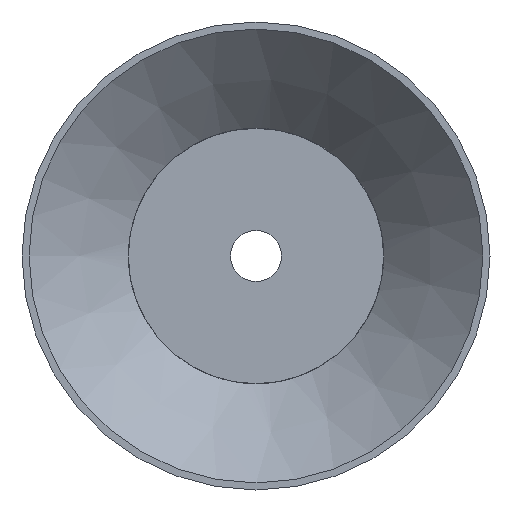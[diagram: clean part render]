
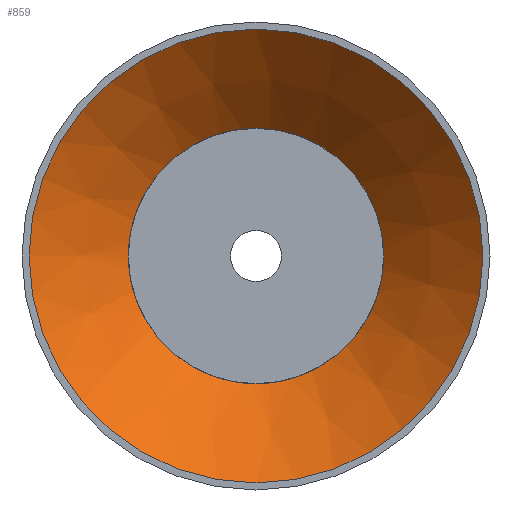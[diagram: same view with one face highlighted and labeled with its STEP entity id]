
A CAD part, front view. The second image highlights one B-rep face of the part: STEP entity #859.
In plain terms, the highlighted conical face has half-angle 45.227 degrees and reference radius 31.679 mm.
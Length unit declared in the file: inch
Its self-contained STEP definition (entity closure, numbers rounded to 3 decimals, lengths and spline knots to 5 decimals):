
#100=(
BOUNDED_CURVE()
B_SPLINE_CURVE(2,(#1197,#1198,#1199),.UNSPECIFIED.,.F.,.F.)
B_SPLINE_CURVE_WITH_KNOTS((3,3),(0.,0.0225),.UNSPECIFIED.)
CURVE()
GEOMETRIC_REPRESENTATION_ITEM()
RATIONAL_B_SPLINE_CURVE((1.,1.,1.))
REPRESENTATION_ITEM('')
);
#101=(
BOUNDED_CURVE()
B_SPLINE_CURVE(2,(#1201,#1202,#1203),.UNSPECIFIED.,.F.,.F.)
B_SPLINE_CURVE_WITH_KNOTS((3,3),(0.84945,0.87196),
 .UNSPECIFIED.)
CURVE()
GEOMETRIC_REPRESENTATION_ITEM()
RATIONAL_B_SPLINE_CURVE((1.,1.,1.))
REPRESENTATION_ITEM('')
);
#102=(
BOUNDED_CURVE()
B_SPLINE_CURVE(2,(#1206,#1207,#1208),.UNSPECIFIED.,.F.,.F.)
B_SPLINE_CURVE_WITH_KNOTS((3,3),(0.,0.0225),.UNSPECIFIED.)
CURVE()
GEOMETRIC_REPRESENTATION_ITEM()
RATIONAL_B_SPLINE_CURVE((1.,1.,1.))
REPRESENTATION_ITEM('')
);
#103=(
BOUNDED_CURVE()
B_SPLINE_CURVE(2,(#1210,#1211,#1212),.UNSPECIFIED.,.F.,.F.)
B_SPLINE_CURVE_WITH_KNOTS((3,3),(0.84929,0.87179),
 .UNSPECIFIED.)
CURVE()
GEOMETRIC_REPRESENTATION_ITEM()
RATIONAL_B_SPLINE_CURVE((1.,1.,1.))
REPRESENTATION_ITEM('')
);
#104=(
BOUNDED_CURVE()
B_SPLINE_CURVE(2,(#1215,#1216,#1217),.UNSPECIFIED.,.F.,.F.)
B_SPLINE_CURVE_WITH_KNOTS((3,3),(0.,0.0225),.UNSPECIFIED.)
CURVE()
GEOMETRIC_REPRESENTATION_ITEM()
RATIONAL_B_SPLINE_CURVE((1.,1.,1.))
REPRESENTATION_ITEM('')
);
#105=(
BOUNDED_CURVE()
B_SPLINE_CURVE(2,(#1219,#1220,#1221),.UNSPECIFIED.,.F.,.F.)
B_SPLINE_CURVE_WITH_KNOTS((3,3),(0.84951,0.87201),
 .UNSPECIFIED.)
CURVE()
GEOMETRIC_REPRESENTATION_ITEM()
RATIONAL_B_SPLINE_CURVE((1.,1.,1.))
REPRESENTATION_ITEM('')
);
#106=(
BOUNDED_CURVE()
B_SPLINE_CURVE(2,(#1224,#1225,#1226),.UNSPECIFIED.,.F.,.F.)
B_SPLINE_CURVE_WITH_KNOTS((3,3),(0.,0.0225),.UNSPECIFIED.)
CURVE()
GEOMETRIC_REPRESENTATION_ITEM()
RATIONAL_B_SPLINE_CURVE((1.,1.,1.))
REPRESENTATION_ITEM('')
);
#107=(
BOUNDED_CURVE()
B_SPLINE_CURVE(2,(#1228,#1229,#1230),.UNSPECIFIED.,.F.,.F.)
B_SPLINE_CURVE_WITH_KNOTS((3,3),(0.8493,0.8718),
 .UNSPECIFIED.)
CURVE()
GEOMETRIC_REPRESENTATION_ITEM()
RATIONAL_B_SPLINE_CURVE((1.,1.,1.))
REPRESENTATION_ITEM('')
);
#128=CONICAL_SURFACE('',#932,1.24721,0.789);
#137=FACE_OUTER_BOUND('',#178,.T.);
#178=EDGE_LOOP('',(#588,#589,#590,#591,#592,#593,#594,#595,#596,#597,#598,
#599,#600,#601,#602,#603,#604,#605,#606,#607,#608));
#223=LINE('',#1194,#253);
#253=VECTOR('',#1037,1.24721);
#279=CIRCLE('',#915,0.89443);
#280=CIRCLE('',#917,0.89443);
#282=CIRCLE('',#920,0.89443);
#285=CIRCLE('',#924,0.89443);
#289=CIRCLE('',#930,1.6);
#290=CIRCLE('',#931,1.6);
#291=CIRCLE('',#933,0.9);
#292=CIRCLE('',#934,0.9);
#293=CIRCLE('',#935,0.9);
#294=CIRCLE('',#936,0.9);
#295=CIRCLE('',#937,0.9);
#315=VERTEX_POINT('',#1145);
#317=VERTEX_POINT('',#1149);
#318=VERTEX_POINT('',#1153);
#320=VERTEX_POINT('',#1156);
#322=VERTEX_POINT('',#1162);
#324=VERTEX_POINT('',#1165);
#327=VERTEX_POINT('',#1172);
#329=VERTEX_POINT('',#1176);
#333=VERTEX_POINT('',#1188);
#334=VERTEX_POINT('',#1189);
#335=VERTEX_POINT('',#1193);
#336=VERTEX_POINT('',#1195);
#337=VERTEX_POINT('',#1200);
#338=VERTEX_POINT('',#1204);
#339=VERTEX_POINT('',#1209);
#340=VERTEX_POINT('',#1213);
#341=VERTEX_POINT('',#1218);
#342=VERTEX_POINT('',#1222);
#343=VERTEX_POINT('',#1227);
#419=EDGE_CURVE('',#317,#315,#279,.T.);
#421=EDGE_CURVE('',#318,#320,#280,.T.);
#425=EDGE_CURVE('',#322,#324,#282,.T.);
#431=EDGE_CURVE('',#329,#327,#285,.T.);
#436=EDGE_CURVE('',#333,#334,#289,.T.);
#437=EDGE_CURVE('',#334,#333,#290,.T.);
#438=EDGE_CURVE('',#334,#335,#223,.T.);
#439=EDGE_CURVE('',#336,#335,#291,.T.);
#440=EDGE_CURVE('',#327,#336,#100,.T.);
#441=EDGE_CURVE('',#337,#329,#101,.T.);
#442=EDGE_CURVE('',#338,#337,#292,.T.);
#443=EDGE_CURVE('',#315,#338,#102,.T.);
#444=EDGE_CURVE('',#339,#317,#103,.T.);
#445=EDGE_CURVE('',#340,#339,#293,.T.);
#446=EDGE_CURVE('',#320,#340,#104,.T.);
#447=EDGE_CURVE('',#341,#318,#105,.T.);
#448=EDGE_CURVE('',#342,#341,#294,.T.);
#449=EDGE_CURVE('',#324,#342,#106,.T.);
#450=EDGE_CURVE('',#343,#322,#107,.T.);
#451=EDGE_CURVE('',#335,#343,#295,.T.);
#588=ORIENTED_EDGE('',*,*,#436,.T.);
#589=ORIENTED_EDGE('',*,*,#438,.T.);
#590=ORIENTED_EDGE('',*,*,#439,.F.);
#591=ORIENTED_EDGE('',*,*,#440,.F.);
#592=ORIENTED_EDGE('',*,*,#431,.F.);
#593=ORIENTED_EDGE('',*,*,#441,.F.);
#594=ORIENTED_EDGE('',*,*,#442,.F.);
#595=ORIENTED_EDGE('',*,*,#443,.F.);
#596=ORIENTED_EDGE('',*,*,#419,.F.);
#597=ORIENTED_EDGE('',*,*,#444,.F.);
#598=ORIENTED_EDGE('',*,*,#445,.F.);
#599=ORIENTED_EDGE('',*,*,#446,.F.);
#600=ORIENTED_EDGE('',*,*,#421,.F.);
#601=ORIENTED_EDGE('',*,*,#447,.F.);
#602=ORIENTED_EDGE('',*,*,#448,.F.);
#603=ORIENTED_EDGE('',*,*,#449,.F.);
#604=ORIENTED_EDGE('',*,*,#425,.F.);
#605=ORIENTED_EDGE('',*,*,#450,.F.);
#606=ORIENTED_EDGE('',*,*,#451,.F.);
#607=ORIENTED_EDGE('',*,*,#438,.F.);
#608=ORIENTED_EDGE('',*,*,#437,.T.);
#859=ADVANCED_FACE('',(#137),#128,.F.);
#915=AXIS2_PLACEMENT_3D('',#1151,#994,#995);
#917=AXIS2_PLACEMENT_3D('',#1157,#999,#1000);
#920=AXIS2_PLACEMENT_3D('',#1166,#1007,#1008);
#924=AXIS2_PLACEMENT_3D('',#1178,#1018,#1019);
#930=AXIS2_PLACEMENT_3D('',#1190,#1031,#1032);
#931=AXIS2_PLACEMENT_3D('',#1191,#1033,#1034);
#932=AXIS2_PLACEMENT_3D('',#1192,#1035,#1036);
#933=AXIS2_PLACEMENT_3D('',#1196,#1038,#1039);
#934=AXIS2_PLACEMENT_3D('',#1205,#1040,#1041);
#935=AXIS2_PLACEMENT_3D('',#1214,#1042,#1043);
#936=AXIS2_PLACEMENT_3D('',#1223,#1044,#1045);
#937=AXIS2_PLACEMENT_3D('',#1231,#1046,#1047);
#994=DIRECTION('center_axis',(0.,-1.,0.));
#995=DIRECTION('ref_axis',(1.,0.,0.));
#999=DIRECTION('center_axis',(0.,-1.,0.));
#1000=DIRECTION('ref_axis',(1.,0.,0.));
#1007=DIRECTION('center_axis',(0.,-1.,0.));
#1008=DIRECTION('ref_axis',(1.,0.,0.));
#1018=DIRECTION('center_axis',(0.,-1.,0.));
#1019=DIRECTION('ref_axis',(1.,0.,0.));
#1031=DIRECTION('center_axis',(0.,-1.,0.));
#1032=DIRECTION('ref_axis',(1.,0.,0.));
#1033=DIRECTION('center_axis',(0.,-1.,0.));
#1034=DIRECTION('ref_axis',(1.,0.,0.));
#1035=DIRECTION('center_axis',(0.,-1.,0.));
#1036=DIRECTION('ref_axis',(1.,0.,0.));
#1037=DIRECTION('',(0.71,0.704,0.));
#1038=DIRECTION('center_axis',(0.,-1.,0.));
#1039=DIRECTION('ref_axis',(1.,0.,0.));
#1040=DIRECTION('center_axis',(0.,-1.,0.));
#1041=DIRECTION('ref_axis',(1.,0.,0.));
#1042=DIRECTION('center_axis',(0.,-1.,0.));
#1043=DIRECTION('ref_axis',(1.,0.,0.));
#1044=DIRECTION('center_axis',(0.,-1.,0.));
#1045=DIRECTION('ref_axis',(1.,0.,0.));
#1046=DIRECTION('center_axis',(0.,-1.,0.));
#1047=DIRECTION('ref_axis',(1.,0.,0.));
#1145=CARTESIAN_POINT('',(0.09993,0.7,0.88883));
#1149=CARTESIAN_POINT('',(0.88882,0.7,0.1));
#1151=CARTESIAN_POINT('Origin',(0.,0.7,0.));
#1153=CARTESIAN_POINT('',(0.09981,0.7,-0.88884));
#1156=CARTESIAN_POINT('',(0.88882,0.7,-0.1));
#1157=CARTESIAN_POINT('Origin',(0.,0.7,0.));
#1162=CARTESIAN_POINT('',(-0.88882,0.7,-0.09999));
#1165=CARTESIAN_POINT('',(-0.1001,0.7,-0.88881));
#1166=CARTESIAN_POINT('Origin',(0.,0.7,0.));
#1172=CARTESIAN_POINT('',(-0.88882,0.7,0.09999));
#1176=CARTESIAN_POINT('',(-0.09986,0.7,0.88884));
#1178=CARTESIAN_POINT('Origin',(0.,0.7,0.));
#1188=CARTESIAN_POINT('',(1.6,0.,0.));
#1189=CARTESIAN_POINT('',(-1.6,0.,0.));
#1190=CARTESIAN_POINT('Origin',(0.,0.,0.));
#1191=CARTESIAN_POINT('Origin',(0.,0.,0.));
#1192=CARTESIAN_POINT('Origin',(0.,0.35,0.));
#1193=CARTESIAN_POINT('',(-0.9,0.69447,0.));
#1194=CARTESIAN_POINT('',(-1.24721,0.35,0.));
#1195=CARTESIAN_POINT('',(-0.89443,0.69447,0.09999));
#1196=CARTESIAN_POINT('Origin',(0.,0.69447,0.));
#1197=CARTESIAN_POINT('Ctrl Pts',(-0.88882,0.7,
0.09999));
#1198=CARTESIAN_POINT('Ctrl Pts',(-0.89162,0.69724,
0.09999));
#1199=CARTESIAN_POINT('Ctrl Pts',(-0.89443,0.69447,
0.09999));
#1200=CARTESIAN_POINT('',(-0.09986,0.69447,0.89444));
#1201=CARTESIAN_POINT('Ctrl Pts',(-0.09986,0.69447,
0.89444));
#1202=CARTESIAN_POINT('Ctrl Pts',(-0.09986,0.69724,
0.89163));
#1203=CARTESIAN_POINT('Ctrl Pts',(-0.09986,0.7,
0.88884));
#1204=CARTESIAN_POINT('',(0.09992,0.69447,0.89444));
#1205=CARTESIAN_POINT('Origin',(0.,0.69447,0.));
#1206=CARTESIAN_POINT('Ctrl Pts',(0.09993,0.7,
0.88883));
#1207=CARTESIAN_POINT('Ctrl Pts',(0.09992,0.69724,0.89162));
#1208=CARTESIAN_POINT('Ctrl Pts',(0.09992,0.69447,
0.89444));
#1209=CARTESIAN_POINT('',(0.89443,0.69447,0.1));
#1210=CARTESIAN_POINT('Ctrl Pts',(0.89443,0.69447,0.1));
#1211=CARTESIAN_POINT('Ctrl Pts',(0.89161,0.69724,0.1));
#1212=CARTESIAN_POINT('Ctrl Pts',(0.88882,0.7,0.1));
#1213=CARTESIAN_POINT('',(0.89443,0.69447,-0.1));
#1214=CARTESIAN_POINT('Origin',(0.,0.69447,0.));
#1215=CARTESIAN_POINT('Ctrl Pts',(0.88882,0.7,-0.1));
#1216=CARTESIAN_POINT('Ctrl Pts',(0.89161,0.69724,-0.1));
#1217=CARTESIAN_POINT('Ctrl Pts',(0.89443,0.69447,-0.1));
#1218=CARTESIAN_POINT('',(0.09981,0.69447,-0.89445));
#1219=CARTESIAN_POINT('Ctrl Pts',(0.09981,0.69447,
-0.89445));
#1220=CARTESIAN_POINT('Ctrl Pts',(0.09981,0.69724,
-0.89164));
#1221=CARTESIAN_POINT('Ctrl Pts',(0.09981,0.7,
-0.88884));
#1222=CARTESIAN_POINT('',(-0.1001,0.69447,-0.89442));
#1223=CARTESIAN_POINT('Origin',(0.,0.69447,0.));
#1224=CARTESIAN_POINT('Ctrl Pts',(-0.1001,0.7,
-0.88881));
#1225=CARTESIAN_POINT('Ctrl Pts',(-0.1001,0.69724,
-0.8916));
#1226=CARTESIAN_POINT('Ctrl Pts',(-0.1001,0.69447,-0.89442));
#1227=CARTESIAN_POINT('',(-0.89443,0.69447,-0.09999));
#1228=CARTESIAN_POINT('Ctrl Pts',(-0.89443,0.69447,
-0.09999));
#1229=CARTESIAN_POINT('Ctrl Pts',(-0.89162,0.69724,
-0.09999));
#1230=CARTESIAN_POINT('Ctrl Pts',(-0.88882,0.7,-0.09999));
#1231=CARTESIAN_POINT('Origin',(0.,0.69447,0.));
